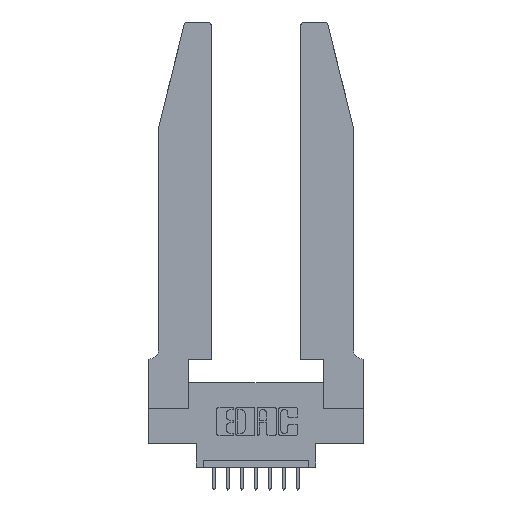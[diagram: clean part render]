
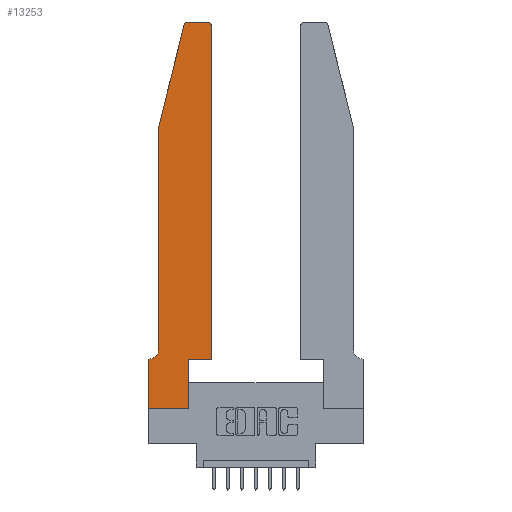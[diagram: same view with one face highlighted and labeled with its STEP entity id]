
A CAD part, top view. The second image highlights one B-rep face of the part: STEP entity #13253.
In plain terms, the highlighted planar face has unit normal (0, 0, 1).
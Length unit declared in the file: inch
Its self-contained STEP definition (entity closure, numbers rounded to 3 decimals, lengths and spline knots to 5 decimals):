
#11 = ORIENTED_EDGE ( 'NONE', *, *, #8745, .T. ) ;
#44 = ORIENTED_EDGE ( 'NONE', *, *, #7376, .T. ) ;
#183 = CARTESIAN_POINT ( 'NONE',  ( 0., 0., 0.37 ) ) ;
#533 = DIRECTION ( 'NONE',  ( 0., -1., 0. ) ) ;
#590 = DIRECTION ( 'NONE',  ( -1., 0., 0. ) ) ;
#843 = DIRECTION ( 'NONE',  ( 0., 0., 1. ) ) ;
#959 = AXIS2_PLACEMENT_3D ( 'NONE', #2659, #6031, #6086 ) ;
#977 = VECTOR ( 'NONE', #1423, 39.37008 ) ;
#1023 = VERTEX_POINT ( 'NONE', #2345 ) ;
#1176 = ORIENTED_EDGE ( 'NONE', *, *, #8492, .T. ) ;
#1192 = LINE ( 'NONE', #8473, #6408 ) ;
#1222 = DIRECTION ( 'NONE',  ( 1., 0., 0. ) ) ;
#1345 = LINE ( 'NONE', #8132, #11615 ) ;
#1423 = DIRECTION ( 'NONE',  ( 1., 0., 0. ) ) ;
#1508 = VECTOR ( 'NONE', #1222, 39.37008 ) ;
#1516 = DIRECTION ( 'NONE',  ( 1., 0., 0. ) ) ;
#1643 = EDGE_CURVE ( 'NONE', #11333, #1023, #10576, .T. ) ;
#1660 = CARTESIAN_POINT ( 'NONE',  ( 0.2605, 2.75, 0.37 ) ) ;
#1713 = LINE ( 'NONE', #8028, #4401 ) ;
#1761 = CARTESIAN_POINT ( 'NONE',  ( 0.0755, 0.35, 0.37 ) ) ;
#1824 = VERTEX_POINT ( 'NONE', #4658 ) ;
#1878 = CARTESIAN_POINT ( 'NONE',  ( 0.0055, 0.42, 0.37 ) ) ;
#1922 = EDGE_CURVE ( 'NONE', #14707, #5411, #1192, .T. ) ;
#1949 = CIRCLE ( 'NONE', #3150, 0.07 ) ;
#2223 = VERTEX_POINT ( 'NONE', #2316 ) ;
#2316 = CARTESIAN_POINT ( 'NONE',  ( 0.4505, 0.35, 0.37 ) ) ;
#2325 = DIRECTION ( 'NONE',  ( 0., -1., 0. ) ) ;
#2345 = CARTESIAN_POINT ( 'NONE',  ( 0.25487, 2.72718, 0.37 ) ) ;
#2589 = LINE ( 'NONE', #12698, #1508 ) ;
#2645 = VECTOR ( 'NONE', #590, 39.37008 ) ;
#2659 = CARTESIAN_POINT ( 'NONE',  ( 0., 0.35, 0.37 ) ) ;
#2796 = EDGE_CURVE ( 'NONE', #1824, #13780, #14357, .T. ) ;
#3150 = AXIS2_PLACEMENT_3D ( 'NONE', #1878, #13369, #4029 ) ;
#3286 = DIRECTION ( 'NONE',  ( 1., 0., 0. ) ) ;
#3365 = ORIENTED_EDGE ( 'NONE', *, *, #1643, .T. ) ;
#3627 = AXIS2_PLACEMENT_3D ( 'NONE', #3765, #13157, #1516 ) ;
#3650 = LINE ( 'NONE', #12372, #5999 ) ;
#3765 = CARTESIAN_POINT ( 'NONE',  ( 0.284, 2.72, 0.37 ) ) ;
#3913 = CARTESIAN_POINT ( 'NONE',  ( 0., 0.35, 0.37 ) ) ;
#4021 = LINE ( 'NONE', #9576, #977 ) ;
#4029 = DIRECTION ( 'NONE',  ( -1., 0., 0. ) ) ;
#4401 = VECTOR ( 'NONE', #9039, 39.37008 ) ;
#4658 = CARTESIAN_POINT ( 'NONE',  ( 0.4505, 2.72, 0.37 ) ) ;
#4855 = ORIENTED_EDGE ( 'NONE', *, *, #13377, .T. ) ;
#4961 = PLANE ( 'NONE',  #959 ) ;
#5282 = VECTOR ( 'NONE', #13196, 39.37008 ) ;
#5411 = VERTEX_POINT ( 'NONE', #183 ) ;
#5721 = VERTEX_POINT ( 'NONE', #11744 ) ;
#5999 = VECTOR ( 'NONE', #9908, 39.37008 ) ;
#6031 = DIRECTION ( 'NONE',  ( 0., 0., 1. ) ) ;
#6075 = ORIENTED_EDGE ( 'NONE', *, *, #14398, .T. ) ;
#6086 = DIRECTION ( 'NONE',  ( 1., 0., 0. ) ) ;
#6374 = LINE ( 'NONE', #1660, #5282 ) ;
#6408 = VECTOR ( 'NONE', #533, 39.37008 ) ;
#6596 = VERTEX_POINT ( 'NONE', #14331 ) ;
#6991 = EDGE_CURVE ( 'NONE', #1023, #10780, #11972, .T. ) ;
#7376 = EDGE_CURVE ( 'NONE', #8371, #2223, #4021, .T. ) ;
#7540 = ORIENTED_EDGE ( 'NONE', *, *, #2796, .T. ) ;
#7603 = EDGE_CURVE ( 'NONE', #5411, #6596, #2589, .T. ) ;
#7613 = ORIENTED_EDGE ( 'NONE', *, *, #1922, .T. ) ;
#7697 = FACE_OUTER_BOUND ( 'NONE', #12449, .T. ) ;
#7752 = CARTESIAN_POINT ( 'NONE',  ( 0.2865, 0.35, 0.37 ) ) ;
#8028 = CARTESIAN_POINT ( 'NONE',  ( 0.2865, 0.35, 0.37 ) ) ;
#8132 = CARTESIAN_POINT ( 'NONE',  ( 0.0755, 2., 0.37 ) ) ;
#8173 = ORIENTED_EDGE ( 'NONE', *, *, #12792, .T. ) ;
#8309 = CARTESIAN_POINT ( 'NONE',  ( 0.0755, 2., 0.37 ) ) ;
#8371 = VERTEX_POINT ( 'NONE', #7752 ) ;
#8463 = ORIENTED_EDGE ( 'NONE', *, *, #6991, .T. ) ;
#8473 = CARTESIAN_POINT ( 'NONE',  ( 0., 0., 0.37 ) ) ;
#8492 = EDGE_CURVE ( 'NONE', #13780, #11333, #6374, .T. ) ;
#8658 = CARTESIAN_POINT ( 'NONE',  ( 0.4205, 2.75, 0.37 ) ) ;
#8745 = EDGE_CURVE ( 'NONE', #2223, #1824, #3650, .T. ) ;
#8901 = ORIENTED_EDGE ( 'NONE', *, *, #7603, .T. ) ;
#9039 = DIRECTION ( 'NONE',  ( 0., 1., 0. ) ) ;
#9576 = CARTESIAN_POINT ( 'NONE',  ( 0.4505, 0.35, 0.37 ) ) ;
#9908 = DIRECTION ( 'NONE',  ( 0., 1., 0. ) ) ;
#10064 = CARTESIAN_POINT ( 'NONE',  ( 0.4205, 2.72, 0.37 ) ) ;
#10576 = CIRCLE ( 'NONE', #3627, 0.03 ) ;
#10780 = VERTEX_POINT ( 'NONE', #8309 ) ;
#10999 = DIRECTION ( 'NONE',  ( -0.239, -0.971, 0. ) ) ;
#11333 = VERTEX_POINT ( 'NONE', #13050 ) ;
#11615 = VECTOR ( 'NONE', #2325, 39.37008 ) ;
#11657 = VERTEX_POINT ( 'NONE', #13504 ) ;
#11744 = CARTESIAN_POINT ( 'NONE',  ( 0.0755, 0.42, 0.37 ) ) ;
#11826 = LINE ( 'NONE', #1761, #2645 ) ;
#11972 = LINE ( 'NONE', #13128, #12885 ) ;
#12372 = CARTESIAN_POINT ( 'NONE',  ( 0.4505, 0.35, 0.37 ) ) ;
#12449 = EDGE_LOOP ( 'NONE', ( #1176, #3365, #8463, #13306, #8173, #4855, #7613, #8901, #6075, #44, #11, #7540 ) ) ;
#12698 = CARTESIAN_POINT ( 'NONE',  ( 0., 0., 0.37 ) ) ;
#12792 = EDGE_CURVE ( 'NONE', #5721, #11657, #1949, .T. ) ;
#12885 = VECTOR ( 'NONE', #10999, 39.37008 ) ;
#13050 = CARTESIAN_POINT ( 'NONE',  ( 0.284, 2.75, 0.37 ) ) ;
#13128 = CARTESIAN_POINT ( 'NONE',  ( 0.0755, 2., 0.37 ) ) ;
#13157 = DIRECTION ( 'NONE',  ( 0., 0., 1. ) ) ;
#13196 = DIRECTION ( 'NONE',  ( -1., 0., 0. ) ) ;
#13253 = ADVANCED_FACE ( 'NONE', ( #7697 ), #4961, .T. ) ;
#13306 = ORIENTED_EDGE ( 'NONE', *, *, #14538, .T. ) ;
#13369 = DIRECTION ( 'NONE',  ( 0., 0., -1. ) ) ;
#13377 = EDGE_CURVE ( 'NONE', #11657, #14707, #11826, .T. ) ;
#13504 = CARTESIAN_POINT ( 'NONE',  ( 0.0055, 0.35, 0.37 ) ) ;
#13780 = VERTEX_POINT ( 'NONE', #8658 ) ;
#14331 = CARTESIAN_POINT ( 'NONE',  ( 0.2865, 0., 0.37 ) ) ;
#14357 = CIRCLE ( 'NONE', #14662, 0.03 ) ;
#14398 = EDGE_CURVE ( 'NONE', #6596, #8371, #1713, .T. ) ;
#14538 = EDGE_CURVE ( 'NONE', #10780, #5721, #1345, .T. ) ;
#14662 = AXIS2_PLACEMENT_3D ( 'NONE', #10064, #843, #3286 ) ;
#14707 = VERTEX_POINT ( 'NONE', #3913 ) ;
